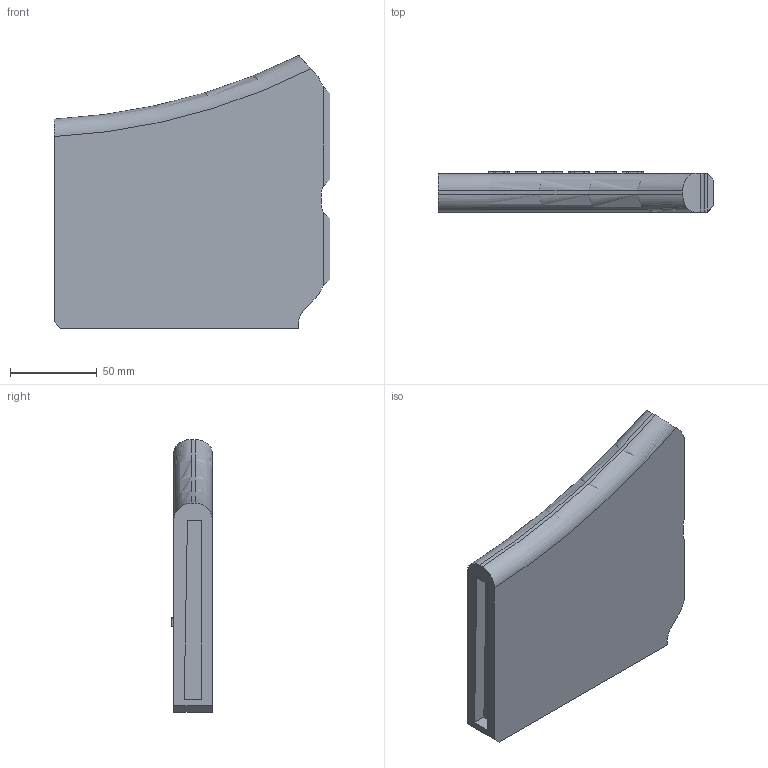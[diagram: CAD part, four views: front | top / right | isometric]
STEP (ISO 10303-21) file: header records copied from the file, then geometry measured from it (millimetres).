
FILE_DESCRIPTION (( 'STEP AP214' ), '1' );
FILE_NAME ('hydrastockx3.STEP', '2013-07-04T02:29:28', ( '' ), ( '' ), 'SwSTEP 2.0', 'SolidWorks 2012', '' );
FILE_SCHEMA (( 'AUTOMOTIVE_DESIGN' ));
Length unit declared in the file: inch
Products named in the file (1): hydrastockx3
Bounding box: 158.99 x 23.51 x 157.29 mm (x, y, z)
Volume: 454443.7 mm3; surface area: 55479.1 mm2
Topology: 1 solids, 1 shells, 126 faces, 334 edges, 220 vertices
Faces by surface type: plane 116, cylinder 8, torus 2
Entity records: 5117 total; most frequent: CARTESIAN_POINT 777, ORIENTED_EDGE 668, DIRECTION 602, EDGE_CURVE 334, LINE 312, VECTOR 312, VERTEX_POINT 220, AXIS2_PLACEMENT_3D 145
